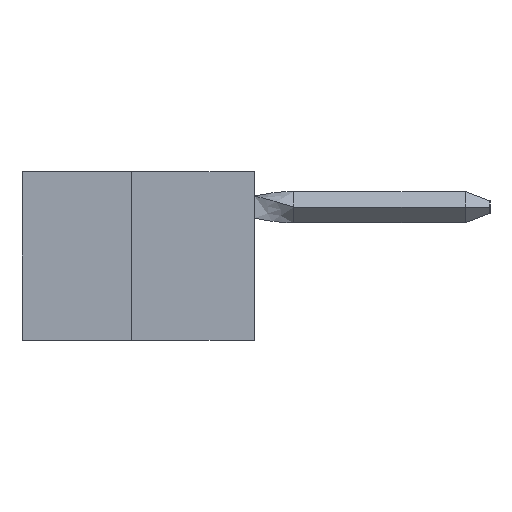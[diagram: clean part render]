
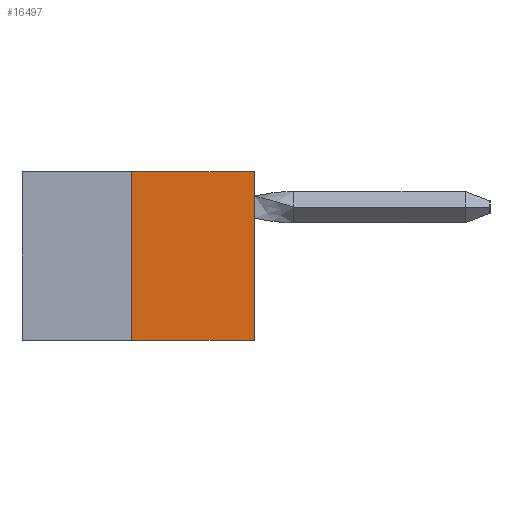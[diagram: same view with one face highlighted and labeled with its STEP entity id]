
A CAD part, left-side view. The second image highlights one B-rep face of the part: STEP entity #16497.
In plain terms, the highlighted planar face has unit normal (-1, 0, 0).
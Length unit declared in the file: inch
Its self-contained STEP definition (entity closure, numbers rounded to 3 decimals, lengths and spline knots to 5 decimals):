
#179 = CARTESIAN_POINT ( 'NONE',  ( 0., 0., 0. ) ) ;
#1231 = VECTOR ( 'NONE', #16057, 39.37008 ) ;
#2131 = EDGE_CURVE ( 'NONE', #13925, #15925, #4074, .T. ) ;
#2148 = LINE ( 'NONE', #7411, #1231 ) ;
#4074 = LINE ( 'NONE', #32471, #17611 ) ;
#4867 = CARTESIAN_POINT ( 'NONE',  ( 0., 0.25, -0.343 ) ) ;
#5675 = EDGE_CURVE ( 'NONE', #13925, #17707, #22980, .T. ) ;
#6066 = PLANE ( 'NONE',  #29254 ) ;
#7411 = CARTESIAN_POINT ( 'NONE',  ( 0., 0.473, 0. ) ) ;
#8666 = CARTESIAN_POINT ( 'NONE',  ( 0., 0.25, 0. ) ) ;
#10360 = EDGE_LOOP ( 'NONE', ( #34937, #22957, #21209, #24351 ) ) ;
#11189 = VERTEX_POINT ( 'NONE', #27564 ) ;
#11323 = DIRECTION ( 'NONE',  ( 0., 0., 1. ) ) ;
#13925 = VERTEX_POINT ( 'NONE', #4867 ) ;
#14641 = DIRECTION ( 'NONE',  ( 0., 0., -1. ) ) ;
#14872 = CARTESIAN_POINT ( 'NONE',  ( 0., 0.473, 0. ) ) ;
#15925 = VERTEX_POINT ( 'NONE', #29191 ) ;
#16057 = DIRECTION ( 'NONE',  ( 0., -1., 0. ) ) ;
#16497 = ADVANCED_FACE ( 'NONE', ( #30395 ), #6066, .F. ) ;
#17611 = VECTOR ( 'NONE', #18049, 39.37008 ) ;
#17707 = VERTEX_POINT ( 'NONE', #20246 ) ;
#18049 = DIRECTION ( 'NONE',  ( 0., -1., 0. ) ) ;
#20125 = VECTOR ( 'NONE', #29084, 39.37008 ) ;
#20246 = CARTESIAN_POINT ( 'NONE',  ( 0., 0.25, 0. ) ) ;
#21209 = ORIENTED_EDGE ( 'NONE', *, *, #2131, .T. ) ;
#22957 = ORIENTED_EDGE ( 'NONE', *, *, #5675, .F. ) ;
#22980 = LINE ( 'NONE', #8666, #25254 ) ;
#24351 = ORIENTED_EDGE ( 'NONE', *, *, #25375, .T. ) ;
#25254 = VECTOR ( 'NONE', #11323, 39.37008 ) ;
#25375 = EDGE_CURVE ( 'NONE', #15925, #11189, #35029, .T. ) ;
#27564 = CARTESIAN_POINT ( 'NONE',  ( 0., 0., 0. ) ) ;
#28380 = DIRECTION ( 'NONE',  ( 1., 0., 0. ) ) ;
#29084 = DIRECTION ( 'NONE',  ( 0., 0., 1. ) ) ;
#29191 = CARTESIAN_POINT ( 'NONE',  ( 0., 0., -0.343 ) ) ;
#29254 = AXIS2_PLACEMENT_3D ( 'NONE', #14872, #28380, #14641 ) ;
#30395 = FACE_OUTER_BOUND ( 'NONE', #10360, .T. ) ;
#32471 = CARTESIAN_POINT ( 'NONE',  ( 0., 0.473, -0.343 ) ) ;
#33263 = EDGE_CURVE ( 'NONE', #17707, #11189, #2148, .T. ) ;
#34937 = ORIENTED_EDGE ( 'NONE', *, *, #33263, .F. ) ;
#35029 = LINE ( 'NONE', #179, #20125 ) ;
